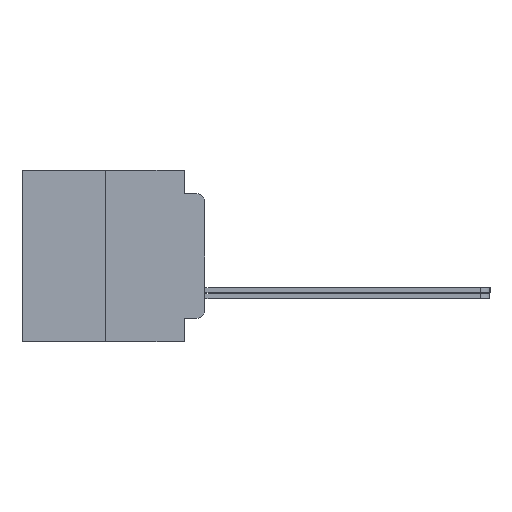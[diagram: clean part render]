
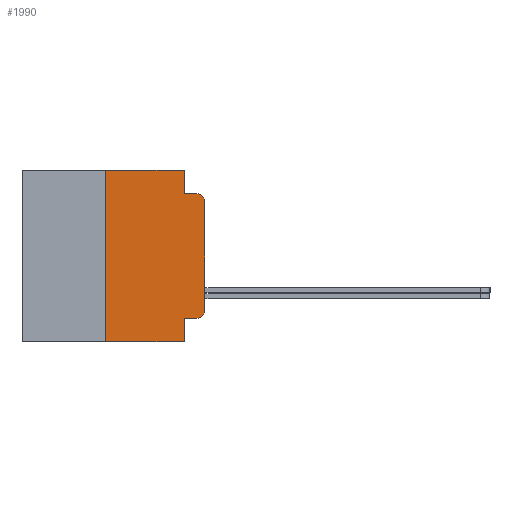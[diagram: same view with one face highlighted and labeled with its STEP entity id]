
A CAD part, left-side view. The second image highlights one B-rep face of the part: STEP entity #1990.
In plain terms, the highlighted planar face has unit normal (-1, 0, 0).
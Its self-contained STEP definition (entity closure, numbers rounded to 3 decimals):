
#270 = CARTESIAN_POINT ( 'NONE',  ( -75.603, 0.508, -3.975 ) ) ;
#691 = CIRCLE ( 'NONE', #5908, 0.508 ) ;
#748 = DIRECTION ( 'NONE',  ( 0., -1., 0. ) ) ;
#1089 = DIRECTION ( 'NONE',  ( 0., 0., 1. ) ) ;
#1462 = LINE ( 'NONE', #22033, #24447 ) ;
#1807 = CARTESIAN_POINT ( 'NONE',  ( -75.603, 6.35, -5.486 ) ) ;
#1990 = ADVANCED_FACE ( 'NONE', ( #20107 ), #23906, .F. ) ;
#2055 = EDGE_CURVE ( 'NONE', #15373, #20506, #1462, .T. ) ;
#2410 = CARTESIAN_POINT ( 'NONE',  ( -75.603, 11.684, 5.486 ) ) ;
#2653 = DIRECTION ( 'NONE',  ( -1., 0., 0. ) ) ;
#2718 = CARTESIAN_POINT ( 'NONE',  ( -75.603, 11.684, 5.486 ) ) ;
#3051 = EDGE_CURVE ( 'NONE', #8847, #20506, #22686, .T. ) ;
#3507 = LINE ( 'NONE', #7449, #10507 ) ;
#3622 = VECTOR ( 'NONE', #1089, 1000. ) ;
#4221 = DIRECTION ( 'NONE',  ( 0., 0., -1. ) ) ;
#4472 = CARTESIAN_POINT ( 'NONE',  ( -75.603, 1.295, 5.486 ) ) ;
#4999 = CARTESIAN_POINT ( 'NONE',  ( -75.603, 1.295, -3.975 ) ) ;
#5045 = VECTOR ( 'NONE', #4221, 1000. ) ;
#5550 = EDGE_CURVE ( 'NONE', #13375, #6227, #7925, .T. ) ;
#5651 = ORIENTED_EDGE ( 'NONE', *, *, #5550, .T. ) ;
#5908 = AXIS2_PLACEMENT_3D ( 'NONE', #20749, #16456, #18604 ) ;
#6225 = VERTEX_POINT ( 'NONE', #15700 ) ;
#6227 = VERTEX_POINT ( 'NONE', #26304 ) ;
#6876 = CARTESIAN_POINT ( 'NONE',  ( -75.603, 0.508, 3.467 ) ) ;
#7129 = ORIENTED_EDGE ( 'NONE', *, *, #3051, .F. ) ;
#7449 = CARTESIAN_POINT ( 'NONE',  ( -75.603, 1.295, 3.975 ) ) ;
#7728 = DIRECTION ( 'NONE',  ( 0., -1., 0. ) ) ;
#7925 = LINE ( 'NONE', #13115, #8914 ) ;
#8847 = VERTEX_POINT ( 'NONE', #4999 ) ;
#8914 = VECTOR ( 'NONE', #23934, 1000. ) ;
#10412 = LINE ( 'NONE', #2718, #20044 ) ;
#10507 = VECTOR ( 'NONE', #7728, 1000. ) ;
#10669 = EDGE_CURVE ( 'NONE', #16177, #15263, #3507, .T. ) ;
#10878 = DIRECTION ( 'NONE',  ( 0., 0., -1. ) ) ;
#11803 = EDGE_CURVE ( 'NONE', #6227, #15263, #16408, .T. ) ;
#12995 = DIRECTION ( 'NONE',  ( 1., 0., 0. ) ) ;
#13115 = CARTESIAN_POINT ( 'NONE',  ( -75.603, 0., 5.486 ) ) ;
#13251 = AXIS2_PLACEMENT_3D ( 'NONE', #6876, #2653, #15377 ) ;
#13375 = VERTEX_POINT ( 'NONE', #23244 ) ;
#13442 = ORIENTED_EDGE ( 'NONE', *, *, #2055, .T. ) ;
#14073 = ORIENTED_EDGE ( 'NONE', *, *, #11803, .T. ) ;
#14100 = ORIENTED_EDGE ( 'NONE', *, *, #24127, .T. ) ;
#14335 = DIRECTION ( 'NONE',  ( 0., 0., -1. ) ) ;
#15195 = DIRECTION ( 'NONE',  ( 0., -1., 0. ) ) ;
#15263 = VERTEX_POINT ( 'NONE', #22742 ) ;
#15373 = VERTEX_POINT ( 'NONE', #1807 ) ;
#15377 = DIRECTION ( 'NONE',  ( 0., 0., -1. ) ) ;
#15636 = EDGE_CURVE ( 'NONE', #6225, #16274, #10412, .T. ) ;
#15700 = CARTESIAN_POINT ( 'NONE',  ( -75.603, 6.35, 5.486 ) ) ;
#15997 = EDGE_CURVE ( 'NONE', #25223, #13375, #691, .T. ) ;
#16177 = VERTEX_POINT ( 'NONE', #25585 ) ;
#16274 = VERTEX_POINT ( 'NONE', #4472 ) ;
#16408 = CIRCLE ( 'NONE', #13251, 0.508 ) ;
#16456 = DIRECTION ( 'NONE',  ( -1., 0., 0. ) ) ;
#17612 = EDGE_CURVE ( 'NONE', #15373, #6225, #19575, .T. ) ;
#17732 = ORIENTED_EDGE ( 'NONE', *, *, #15997, .T. ) ;
#18088 = AXIS2_PLACEMENT_3D ( 'NONE', #2410, #12995, #10878 ) ;
#18604 = DIRECTION ( 'NONE',  ( 0., 0., -1. ) ) ;
#18732 = CARTESIAN_POINT ( 'NONE',  ( -75.603, 1.295, 0. ) ) ;
#18946 = LINE ( 'NONE', #18732, #19944 ) ;
#19575 = LINE ( 'NONE', #22128, #3622 ) ;
#19586 = CARTESIAN_POINT ( 'NONE',  ( -75.603, 1.295, -3.975 ) ) ;
#19898 = EDGE_LOOP ( 'NONE', ( #14100, #17732, #5651, #14073, #20355, #22072, #27290, #23001, #13442, #7129 ) ) ;
#19944 = VECTOR ( 'NONE', #14335, 1000. ) ;
#20033 = CARTESIAN_POINT ( 'NONE',  ( -75.603, 1.295, -5.486 ) ) ;
#20044 = VECTOR ( 'NONE', #748, 1000. ) ;
#20107 = FACE_OUTER_BOUND ( 'NONE', #19898, .T. ) ;
#20355 = ORIENTED_EDGE ( 'NONE', *, *, #10669, .F. ) ;
#20506 = VERTEX_POINT ( 'NONE', #20033 ) ;
#20749 = CARTESIAN_POINT ( 'NONE',  ( -75.603, 0.508, -3.467 ) ) ;
#21244 = CARTESIAN_POINT ( 'NONE',  ( -75.603, 1.295, 0. ) ) ;
#22033 = CARTESIAN_POINT ( 'NONE',  ( -75.603, 11.684, -5.486 ) ) ;
#22058 = LINE ( 'NONE', #19586, #26676 ) ;
#22072 = ORIENTED_EDGE ( 'NONE', *, *, #26507, .F. ) ;
#22128 = CARTESIAN_POINT ( 'NONE',  ( -75.603, 6.35, -5.486 ) ) ;
#22686 = LINE ( 'NONE', #21244, #5045 ) ;
#22742 = CARTESIAN_POINT ( 'NONE',  ( -75.603, 0.508, 3.975 ) ) ;
#23001 = ORIENTED_EDGE ( 'NONE', *, *, #17612, .F. ) ;
#23244 = CARTESIAN_POINT ( 'NONE',  ( -75.603, 0., -3.467 ) ) ;
#23906 = PLANE ( 'NONE',  #18088 ) ;
#23934 = DIRECTION ( 'NONE',  ( 0., 0., 1. ) ) ;
#24127 = EDGE_CURVE ( 'NONE', #8847, #25223, #22058, .T. ) ;
#24182 = DIRECTION ( 'NONE',  ( 0., -1., 0. ) ) ;
#24447 = VECTOR ( 'NONE', #24182, 1000. ) ;
#25223 = VERTEX_POINT ( 'NONE', #270 ) ;
#25585 = CARTESIAN_POINT ( 'NONE',  ( -75.603, 1.295, 3.975 ) ) ;
#26304 = CARTESIAN_POINT ( 'NONE',  ( -75.603, 0., 3.467 ) ) ;
#26507 = EDGE_CURVE ( 'NONE', #16274, #16177, #18946, .T. ) ;
#26676 = VECTOR ( 'NONE', #15195, 1000. ) ;
#27290 = ORIENTED_EDGE ( 'NONE', *, *, #15636, .F. ) ;
